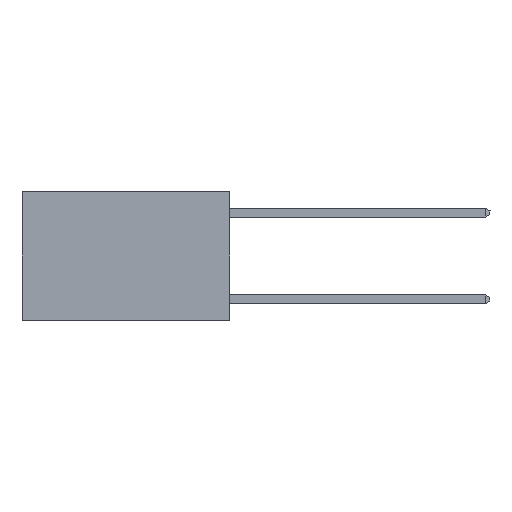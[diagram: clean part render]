
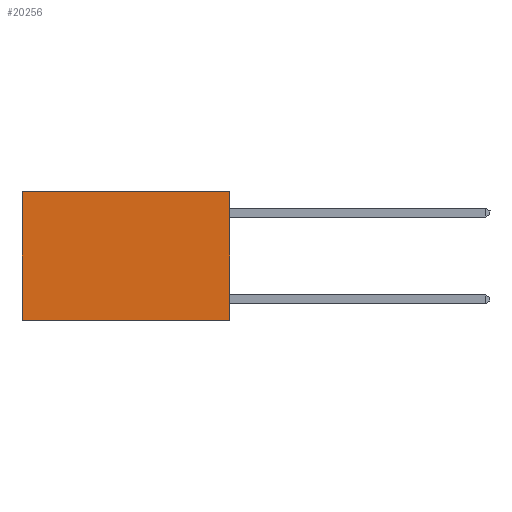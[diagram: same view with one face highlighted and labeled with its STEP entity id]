
A CAD part, left-side view. The second image highlights one B-rep face of the part: STEP entity #20256.
In plain terms, the highlighted planar face has unit normal (-1, 0, 0).
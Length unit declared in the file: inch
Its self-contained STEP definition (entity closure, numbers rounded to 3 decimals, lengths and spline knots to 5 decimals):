
#595 = CARTESIAN_POINT ( 'NONE',  ( 0.2625, 0.6, -0.37 ) ) ;
#1571 = LINE ( 'NONE', #13975, #18406 ) ;
#1952 = ORIENTED_EDGE ( 'NONE', *, *, #3300, .T. ) ;
#2074 = DIRECTION ( 'NONE',  ( 0., 1., 0. ) ) ;
#2119 = CARTESIAN_POINT ( 'NONE',  ( 0.2625, 0.6, 0. ) ) ;
#2938 = VERTEX_POINT ( 'NONE', #10168 ) ;
#3037 = VECTOR ( 'NONE', #12699, 39.37008 ) ;
#3194 = CARTESIAN_POINT ( 'NONE',  ( 0.2625, 0., -0.37 ) ) ;
#3300 = EDGE_CURVE ( 'NONE', #15748, #16823, #1571, .T. ) ;
#4177 = ORIENTED_EDGE ( 'NONE', *, *, #4660, .F. ) ;
#4660 = EDGE_CURVE ( 'NONE', #20955, #2938, #9478, .T. ) ;
#4670 = CARTESIAN_POINT ( 'NONE',  ( 0.2625, 0., 0. ) ) ;
#4737 = EDGE_LOOP ( 'NONE', ( #1952, #20633, #4177, #7326 ) ) ;
#7326 = ORIENTED_EDGE ( 'NONE', *, *, #12247, .T. ) ;
#9478 = LINE ( 'NONE', #19607, #3037 ) ;
#10168 = CARTESIAN_POINT ( 'NONE',  ( 0.2625, 0., -0.37 ) ) ;
#11880 = PLANE ( 'NONE',  #18606 ) ;
#12204 = VECTOR ( 'NONE', #14970, 39.37008 ) ;
#12247 = EDGE_CURVE ( 'NONE', #20955, #15748, #15858, .T. ) ;
#12699 = DIRECTION ( 'NONE',  ( 0., 0., -1. ) ) ;
#13135 = FACE_OUTER_BOUND ( 'NONE', #4737, .T. ) ;
#13975 = CARTESIAN_POINT ( 'NONE',  ( 0.2625, 0.6, 0. ) ) ;
#14970 = DIRECTION ( 'NONE',  ( 0., 1., 0. ) ) ;
#15676 = CARTESIAN_POINT ( 'NONE',  ( 0.2625, 0., 0. ) ) ;
#15748 = VERTEX_POINT ( 'NONE', #2119 ) ;
#15858 = LINE ( 'NONE', #20536, #16539 ) ;
#16539 = VECTOR ( 'NONE', #2074, 39.37008 ) ;
#16653 = LINE ( 'NONE', #3194, #12204 ) ;
#16823 = VERTEX_POINT ( 'NONE', #595 ) ;
#17320 = DIRECTION ( 'NONE',  ( 0., 0., -1. ) ) ;
#18406 = VECTOR ( 'NONE', #17320, 39.37008 ) ;
#18606 = AXIS2_PLACEMENT_3D ( 'NONE', #4670, #21604, #21938 ) ;
#19607 = CARTESIAN_POINT ( 'NONE',  ( 0.2625, 0., 0. ) ) ;
#19763 = EDGE_CURVE ( 'NONE', #2938, #16823, #16653, .T. ) ;
#20256 = ADVANCED_FACE ( 'NONE', ( #13135 ), #11880, .F. ) ;
#20536 = CARTESIAN_POINT ( 'NONE',  ( 0.2625, 0., 0. ) ) ;
#20633 = ORIENTED_EDGE ( 'NONE', *, *, #19763, .F. ) ;
#20955 = VERTEX_POINT ( 'NONE', #15676 ) ;
#21604 = DIRECTION ( 'NONE',  ( 1., 0., 0. ) ) ;
#21938 = DIRECTION ( 'NONE',  ( 0., 0., -1. ) ) ;
